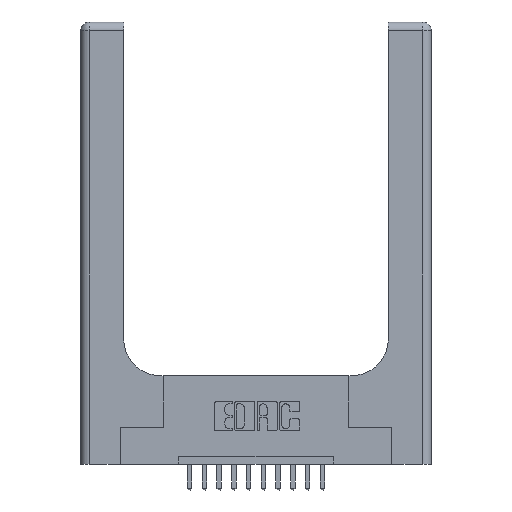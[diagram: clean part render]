
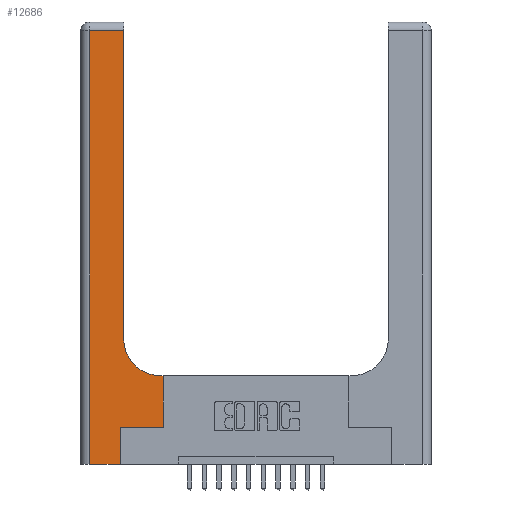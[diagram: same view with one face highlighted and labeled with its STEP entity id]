
A CAD part, top view. The second image highlights one B-rep face of the part: STEP entity #12686.
In plain terms, the highlighted planar face has unit normal (0, 0, 1).
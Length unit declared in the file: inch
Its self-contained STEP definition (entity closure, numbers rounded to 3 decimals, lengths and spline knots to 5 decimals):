
#103 = AXIS2_PLACEMENT_3D ( 'NONE', #5761, #2001, #15141 ) ;
#143 = CARTESIAN_POINT ( 'NONE',  ( 0.06, 2.94, 0.37 ) ) ;
#192 = VERTEX_POINT ( 'NONE', #9629 ) ;
#474 = CARTESIAN_POINT ( 'NONE',  ( 0.2915, 0.85, 0.37 ) ) ;
#846 = EDGE_CURVE ( 'NONE', #6539, #9341, #13525, .T. ) ;
#978 = EDGE_CURVE ( 'NONE', #16103, #16634, #14950, .T. ) ;
#1042 = ORIENTED_EDGE ( 'NONE', *, *, #2332, .T. ) ;
#1082 = DIRECTION ( 'NONE',  ( 1., 0., 0. ) ) ;
#1369 = CARTESIAN_POINT ( 'NONE',  ( 0.06, 3., 0.37 ) ) ;
#1457 = VERTEX_POINT ( 'NONE', #6530 ) ;
#1555 = CARTESIAN_POINT ( 'NONE',  ( 0.06, 0., 0.37 ) ) ;
#1725 = VECTOR ( 'NONE', #2906, 39.37008 ) ;
#1895 = VERTEX_POINT ( 'NONE', #474 ) ;
#1996 = VECTOR ( 'NONE', #8707, 39.37008 ) ;
#2001 = DIRECTION ( 'NONE',  ( 0., 0., -1. ) ) ;
#2163 = VECTOR ( 'NONE', #7127, 39.37008 ) ;
#2199 = CARTESIAN_POINT ( 'NONE',  ( 0.5585, 0.25, 0.37 ) ) ;
#2249 = CIRCLE ( 'NONE', #13205, 0.25 ) ;
#2332 = EDGE_CURVE ( 'NONE', #1895, #14425, #16992, .T. ) ;
#2431 = LINE ( 'NONE', #15031, #10080 ) ;
#2619 = ORIENTED_EDGE ( 'NONE', *, *, #846, .T. ) ;
#2906 = DIRECTION ( 'NONE',  ( 0., -1., 0. ) ) ;
#3484 = ORIENTED_EDGE ( 'NONE', *, *, #8212, .T. ) ;
#3907 = CARTESIAN_POINT ( 'NONE',  ( 0.269, 0.25, 0.37 ) ) ;
#3973 = VECTOR ( 'NONE', #9731, 39.37008 ) ;
#4149 = DIRECTION ( 'NONE',  ( 1., 0., 0. ) ) ;
#4328 = ORIENTED_EDGE ( 'NONE', *, *, #10815, .T. ) ;
#4537 = DIRECTION ( 'NONE',  ( -1., 0., 0. ) ) ;
#4779 = CARTESIAN_POINT ( 'NONE',  ( 0.2915, 2.94, 0.37 ) ) ;
#4895 = LINE ( 'NONE', #5580, #1996 ) ;
#5058 = EDGE_CURVE ( 'NONE', #192, #1457, #15619, .T. ) ;
#5530 = DIRECTION ( 'NONE',  ( -1., 0., 0. ) ) ;
#5580 = CARTESIAN_POINT ( 'NONE',  ( 0., 0., 0.37 ) ) ;
#5761 = CARTESIAN_POINT ( 'NONE',  ( 0., 3., 0.37 ) ) ;
#5911 = VERTEX_POINT ( 'NONE', #13611 ) ;
#5925 = EDGE_LOOP ( 'NONE', ( #1042, #3484, #7921, #7239, #2619, #4328, #13825, #6055, #16136 ) ) ;
#6053 = EDGE_CURVE ( 'NONE', #16634, #6539, #4895, .T. ) ;
#6055 = ORIENTED_EDGE ( 'NONE', *, *, #9086, .T. ) ;
#6530 = CARTESIAN_POINT ( 'NONE',  ( 0.5585, 0.6, 0.37 ) ) ;
#6539 = VERTEX_POINT ( 'NONE', #9032 ) ;
#6923 = LINE ( 'NONE', #10783, #16179 ) ;
#7127 = DIRECTION ( 'NONE',  ( 0., 1., 0. ) ) ;
#7239 = ORIENTED_EDGE ( 'NONE', *, *, #6053, .T. ) ;
#7921 = ORIENTED_EDGE ( 'NONE', *, *, #978, .T. ) ;
#8212 = EDGE_CURVE ( 'NONE', #14425, #16103, #2431, .T. ) ;
#8265 = CARTESIAN_POINT ( 'NONE',  ( 0.2915, 0.6, 0.37 ) ) ;
#8620 = CARTESIAN_POINT ( 'NONE',  ( 0.269, 0., 0.37 ) ) ;
#8707 = DIRECTION ( 'NONE',  ( 1., 0., 0. ) ) ;
#9032 = CARTESIAN_POINT ( 'NONE',  ( 0.269, 0., 0.37 ) ) ;
#9086 = EDGE_CURVE ( 'NONE', #1457, #5911, #9670, .T. ) ;
#9146 = DIRECTION ( 'NONE',  ( 0., 0., -1. ) ) ;
#9341 = VERTEX_POINT ( 'NONE', #3907 ) ;
#9629 = CARTESIAN_POINT ( 'NONE',  ( 0.5585, 0.25, 0.37 ) ) ;
#9670 = LINE ( 'NONE', #8265, #16259 ) ;
#9731 = DIRECTION ( 'NONE',  ( 0., 1., 0. ) ) ;
#10080 = VECTOR ( 'NONE', #4537, 39.37008 ) ;
#10759 = FACE_OUTER_BOUND ( 'NONE', #5925, .T. ) ;
#10783 = CARTESIAN_POINT ( 'NONE',  ( 0.269, 0.25, 0.37 ) ) ;
#10815 = EDGE_CURVE ( 'NONE', #9341, #192, #6923, .T. ) ;
#10937 = CARTESIAN_POINT ( 'NONE',  ( 0.2915, 3., 0.37 ) ) ;
#12567 = PLANE ( 'NONE',  #103 ) ;
#12686 = ADVANCED_FACE ( 'NONE', ( #10759 ), #12567, .F. ) ;
#12959 = VECTOR ( 'NONE', #16648, 39.37008 ) ;
#13205 = AXIS2_PLACEMENT_3D ( 'NONE', #14317, #9146, #1082 ) ;
#13525 = LINE ( 'NONE', #8620, #2163 ) ;
#13611 = CARTESIAN_POINT ( 'NONE',  ( 0.5415, 0.6, 0.37 ) ) ;
#13825 = ORIENTED_EDGE ( 'NONE', *, *, #5058, .T. ) ;
#14043 = EDGE_CURVE ( 'NONE', #5911, #1895, #2249, .T. ) ;
#14317 = CARTESIAN_POINT ( 'NONE',  ( 0.5415, 0.85, 0.37 ) ) ;
#14425 = VERTEX_POINT ( 'NONE', #4779 ) ;
#14950 = LINE ( 'NONE', #1369, #1725 ) ;
#15031 = CARTESIAN_POINT ( 'NONE',  ( 0., 2.94, 0.37 ) ) ;
#15141 = DIRECTION ( 'NONE',  ( -1., 0., 0. ) ) ;
#15619 = LINE ( 'NONE', #2199, #12959 ) ;
#16103 = VERTEX_POINT ( 'NONE', #143 ) ;
#16136 = ORIENTED_EDGE ( 'NONE', *, *, #14043, .T. ) ;
#16179 = VECTOR ( 'NONE', #4149, 39.37008 ) ;
#16259 = VECTOR ( 'NONE', #5530, 39.37008 ) ;
#16634 = VERTEX_POINT ( 'NONE', #1555 ) ;
#16648 = DIRECTION ( 'NONE',  ( 0., 1., 0. ) ) ;
#16992 = LINE ( 'NONE', #10937, #3973 ) ;
